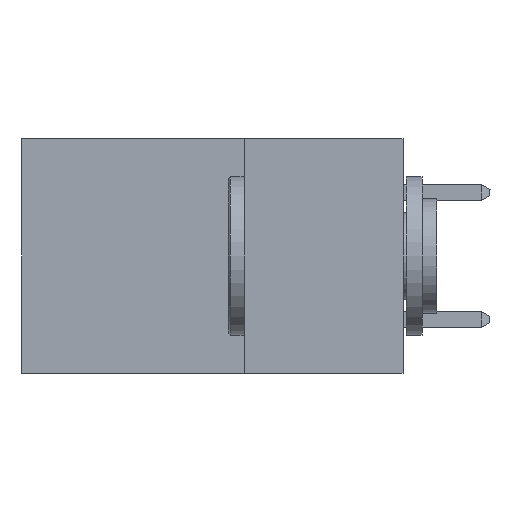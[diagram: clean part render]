
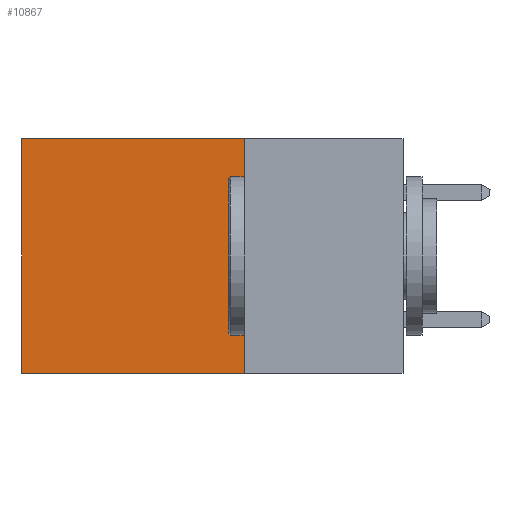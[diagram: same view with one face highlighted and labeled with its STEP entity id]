
A CAD part, left-side view. The second image highlights one B-rep face of the part: STEP entity #10867.
In plain terms, the highlighted planar face has unit normal (-1, 0, 0).
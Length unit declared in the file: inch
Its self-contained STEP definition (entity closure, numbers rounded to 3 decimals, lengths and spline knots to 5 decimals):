
#198 = AXIS2_PLACEMENT_3D ( 'NONE', #18646, #7022, #20591 ) ;
#353 = EDGE_CURVE ( 'NONE', #827, #447, #11065, .T. ) ;
#447 = VERTEX_POINT ( 'NONE', #15509 ) ;
#827 = VERTEX_POINT ( 'NONE', #9485 ) ;
#1340 = DIRECTION ( 'NONE',  ( 0., 0., -1. ) ) ;
#2252 = FACE_OUTER_BOUND ( 'NONE', #23817, .T. ) ;
#3929 = EDGE_CURVE ( 'NONE', #21432, #827, #19720, .T. ) ;
#4217 = CARTESIAN_POINT ( 'NONE',  ( 0.2875, 0.25, -0.37 ) ) ;
#4248 = VECTOR ( 'NONE', #1340, 39.37008 ) ;
#5021 = CARTESIAN_POINT ( 'NONE',  ( 0.2875, 0.6, 0. ) ) ;
#6571 = ORIENTED_EDGE ( 'NONE', *, *, #19413, .T. ) ;
#7022 = DIRECTION ( 'NONE',  ( 1., 0., 0. ) ) ;
#7109 = DIRECTION ( 'NONE',  ( 0., 1., 0. ) ) ;
#8909 = VERTEX_POINT ( 'NONE', #5021 ) ;
#9485 = CARTESIAN_POINT ( 'NONE',  ( 0.2875, 0.25, -0.37 ) ) ;
#10484 = VECTOR ( 'NONE', #7109, 39.37008 ) ;
#10867 = ADVANCED_FACE ( 'NONE', ( #2252 ), #24273, .F. ) ;
#11065 = LINE ( 'NONE', #4217, #10484 ) ;
#11722 = ORIENTED_EDGE ( 'NONE', *, *, #23343, .T. ) ;
#12260 = LINE ( 'NONE', #16447, #17433 ) ;
#12554 = DIRECTION ( 'NONE',  ( 0., 0., -1. ) ) ;
#15509 = CARTESIAN_POINT ( 'NONE',  ( 0.2875, 0.6, -0.37 ) ) ;
#16447 = CARTESIAN_POINT ( 'NONE',  ( 0.2875, 0.6, 0. ) ) ;
#16955 = LINE ( 'NONE', #17569, #22093 ) ;
#17433 = VECTOR ( 'NONE', #12554, 39.37008 ) ;
#17569 = CARTESIAN_POINT ( 'NONE',  ( 0.2875, 0.25, 0. ) ) ;
#17770 = ORIENTED_EDGE ( 'NONE', *, *, #353, .F. ) ;
#18646 = CARTESIAN_POINT ( 'NONE',  ( 0.2875, 0.25, 0. ) ) ;
#18831 = ORIENTED_EDGE ( 'NONE', *, *, #3929, .F. ) ;
#19413 = EDGE_CURVE ( 'NONE', #8909, #447, #12260, .T. ) ;
#19720 = LINE ( 'NONE', #24587, #4248 ) ;
#20591 = DIRECTION ( 'NONE',  ( 0., 0., -1. ) ) ;
#21432 = VERTEX_POINT ( 'NONE', #24337 ) ;
#22093 = VECTOR ( 'NONE', #23284, 39.37008 ) ;
#23284 = DIRECTION ( 'NONE',  ( 0., 1., 0. ) ) ;
#23343 = EDGE_CURVE ( 'NONE', #21432, #8909, #16955, .T. ) ;
#23817 = EDGE_LOOP ( 'NONE', ( #6571, #17770, #18831, #11722 ) ) ;
#24273 = PLANE ( 'NONE',  #198 ) ;
#24337 = CARTESIAN_POINT ( 'NONE',  ( 0.2875, 0.25, 0. ) ) ;
#24587 = CARTESIAN_POINT ( 'NONE',  ( 0.2875, 0.25, 0. ) ) ;
